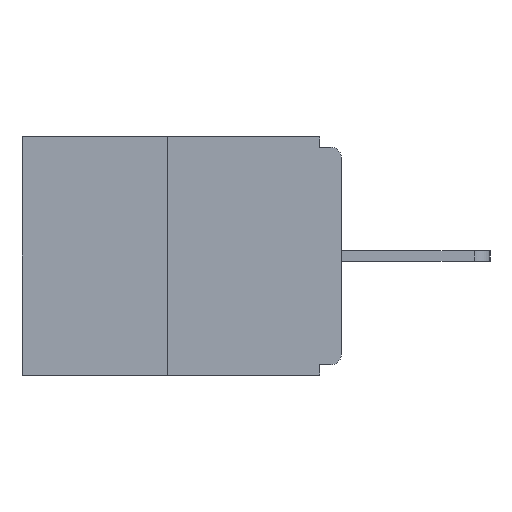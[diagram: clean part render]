
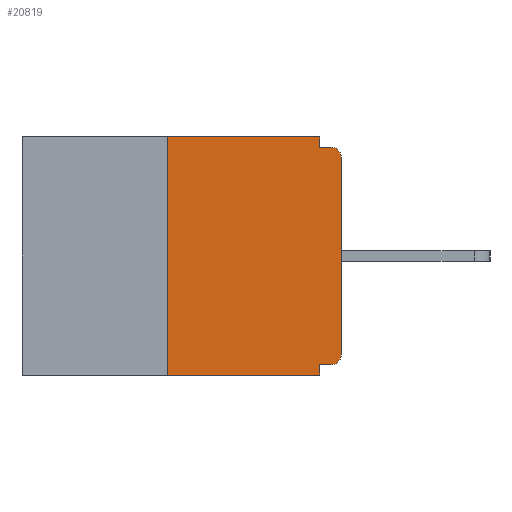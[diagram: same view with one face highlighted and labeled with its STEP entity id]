
A CAD part, left-side view. The second image highlights one B-rep face of the part: STEP entity #20819.
In plain terms, the highlighted planar face has unit normal (-1, 0, 0).
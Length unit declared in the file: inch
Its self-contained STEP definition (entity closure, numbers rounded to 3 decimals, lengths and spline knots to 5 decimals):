
#95 = DIRECTION ( 'NONE',  ( -1., 0., 0. ) ) ;
#302 = EDGE_CURVE ( 'NONE', #7137, #6968, #13642, .T. ) ;
#797 = DIRECTION ( 'NONE',  ( 0., 1., 0. ) ) ;
#963 = ORIENTED_EDGE ( 'NONE', *, *, #16345, .F. ) ;
#1202 = PLANE ( 'NONE',  #10580 ) ;
#1328 = DIRECTION ( 'NONE',  ( 0., 0., -1. ) ) ;
#1522 = CARTESIAN_POINT ( 'NONE',  ( 0., 0.46, 0. ) ) ;
#1648 = VERTEX_POINT ( 'NONE', #4139 ) ;
#1954 = EDGE_CURVE ( 'NONE', #13707, #7137, #19264, .T. ) ;
#2120 = DIRECTION ( 'NONE',  ( 0., -1., 0. ) ) ;
#2138 = VECTOR ( 'NONE', #10817, 39.37008 ) ;
#2271 = CARTESIAN_POINT ( 'NONE',  ( 0., 0.25, 0. ) ) ;
#2463 = CARTESIAN_POINT ( 'NONE',  ( 0., 0.031, 0. ) ) ;
#3085 = DIRECTION ( 'NONE',  ( 0., -1., 0. ) ) ;
#3552 = CARTESIAN_POINT ( 'NONE',  ( 0., 0.46, -0.343 ) ) ;
#3755 = CARTESIAN_POINT ( 'NONE',  ( 0., 0.25, 0. ) ) ;
#4139 = CARTESIAN_POINT ( 'NONE',  ( 0., 0.015, -0.328 ) ) ;
#4356 = DIRECTION ( 'NONE',  ( 0., 0., -1. ) ) ;
#4429 = CARTESIAN_POINT ( 'NONE',  ( 0., 0.031, -0.343 ) ) ;
#4541 = VECTOR ( 'NONE', #20364, 39.37008 ) ;
#4581 = LINE ( 'NONE', #11213, #12436 ) ;
#4691 = CARTESIAN_POINT ( 'NONE',  ( 0., 0.46, 0. ) ) ;
#4740 = AXIS2_PLACEMENT_3D ( 'NONE', #11825, #95, #13228 ) ;
#5364 = ORIENTED_EDGE ( 'NONE', *, *, #1954, .F. ) ;
#5412 = ORIENTED_EDGE ( 'NONE', *, *, #21240, .F. ) ;
#5984 = ORIENTED_EDGE ( 'NONE', *, *, #302, .F. ) ;
#6381 = VERTEX_POINT ( 'NONE', #8549 ) ;
#6968 = VERTEX_POINT ( 'NONE', #12959 ) ;
#7137 = VERTEX_POINT ( 'NONE', #11759 ) ;
#8549 = CARTESIAN_POINT ( 'NONE',  ( 0., 0., -0.03 ) ) ;
#8566 = DIRECTION ( 'NONE',  ( -1., 0., 0. ) ) ;
#8601 = ORIENTED_EDGE ( 'NONE', *, *, #15898, .T. ) ;
#8761 = CARTESIAN_POINT ( 'NONE',  ( 0., 0.031, -0.328 ) ) ;
#8878 = DIRECTION ( 'NONE',  ( 0., 0., 1. ) ) ;
#8931 = CARTESIAN_POINT ( 'NONE',  ( 0., 0., -0.328 ) ) ;
#9085 = CARTESIAN_POINT ( 'NONE',  ( 0., 0., -0.313 ) ) ;
#9409 = CARTESIAN_POINT ( 'NONE',  ( 0., 0., 0. ) ) ;
#9641 = EDGE_CURVE ( 'NONE', #6381, #6968, #14069, .T. ) ;
#9679 = EDGE_CURVE ( 'NONE', #1648, #11336, #13044, .T. ) ;
#9800 = CARTESIAN_POINT ( 'NONE',  ( 0., 0.031, 0. ) ) ;
#9898 = VECTOR ( 'NONE', #16007, 39.37008 ) ;
#9943 = LINE ( 'NONE', #3552, #18592 ) ;
#10031 = EDGE_CURVE ( 'NONE', #11819, #18673, #9943, .T. ) ;
#10580 = AXIS2_PLACEMENT_3D ( 'NONE', #1522, #20942, #4356 ) ;
#10817 = DIRECTION ( 'NONE',  ( 0., 0., 1. ) ) ;
#11213 = CARTESIAN_POINT ( 'NONE',  ( 0., 0.031, -0.343 ) ) ;
#11247 = VERTEX_POINT ( 'NONE', #8761 ) ;
#11336 = VERTEX_POINT ( 'NONE', #9085 ) ;
#11759 = CARTESIAN_POINT ( 'NONE',  ( 0., 0.031, -0.015 ) ) ;
#11819 = VERTEX_POINT ( 'NONE', #14136 ) ;
#11825 = CARTESIAN_POINT ( 'NONE',  ( 0., 0.015, -0.03 ) ) ;
#12436 = VECTOR ( 'NONE', #1328, 39.37008 ) ;
#12959 = CARTESIAN_POINT ( 'NONE',  ( 0., 0.015, -0.015 ) ) ;
#12971 = VECTOR ( 'NONE', #3085, 39.37008 ) ;
#13044 = CIRCLE ( 'NONE', #15822, 0.015 ) ;
#13228 = DIRECTION ( 'NONE',  ( 0., 0., -1. ) ) ;
#13495 = EDGE_LOOP ( 'NONE', ( #16541, #5412, #16545, #14215, #963, #18309, #8601, #16859, #5984, #5364 ) ) ;
#13642 = LINE ( 'NONE', #20262, #4541 ) ;
#13707 = VERTEX_POINT ( 'NONE', #9800 ) ;
#13778 = EDGE_CURVE ( 'NONE', #11247, #18673, #4581, .T. ) ;
#14069 = CIRCLE ( 'NONE', #4740, 0.015 ) ;
#14136 = CARTESIAN_POINT ( 'NONE',  ( 0., 0.25, -0.343 ) ) ;
#14215 = ORIENTED_EDGE ( 'NONE', *, *, #13778, .F. ) ;
#14265 = VECTOR ( 'NONE', #797, 39.37008 ) ;
#15605 = LINE ( 'NONE', #2271, #17277 ) ;
#15822 = AXIS2_PLACEMENT_3D ( 'NONE', #18435, #8566, #21275 ) ;
#15898 = EDGE_CURVE ( 'NONE', #11336, #6381, #18935, .T. ) ;
#16007 = DIRECTION ( 'NONE',  ( 0., 0., -1. ) ) ;
#16345 = EDGE_CURVE ( 'NONE', #1648, #11247, #20423, .T. ) ;
#16541 = ORIENTED_EDGE ( 'NONE', *, *, #20534, .F. ) ;
#16545 = ORIENTED_EDGE ( 'NONE', *, *, #10031, .T. ) ;
#16859 = ORIENTED_EDGE ( 'NONE', *, *, #9641, .T. ) ;
#17277 = VECTOR ( 'NONE', #8878, 39.37008 ) ;
#17450 = VERTEX_POINT ( 'NONE', #3755 ) ;
#18309 = ORIENTED_EDGE ( 'NONE', *, *, #9679, .T. ) ;
#18435 = CARTESIAN_POINT ( 'NONE',  ( 0., 0.015, -0.313 ) ) ;
#18592 = VECTOR ( 'NONE', #2120, 39.37008 ) ;
#18673 = VERTEX_POINT ( 'NONE', #4429 ) ;
#18935 = LINE ( 'NONE', #9409, #2138 ) ;
#19264 = LINE ( 'NONE', #2463, #9898 ) ;
#19560 = LINE ( 'NONE', #4691, #12971 ) ;
#20262 = CARTESIAN_POINT ( 'NONE',  ( 0., 0., -0.015 ) ) ;
#20364 = DIRECTION ( 'NONE',  ( 0., -1., 0. ) ) ;
#20423 = LINE ( 'NONE', #8931, #14265 ) ;
#20534 = EDGE_CURVE ( 'NONE', #17450, #13707, #19560, .T. ) ;
#20613 = FACE_OUTER_BOUND ( 'NONE', #13495, .T. ) ;
#20819 = ADVANCED_FACE ( 'NONE', ( #20613 ), #1202, .F. ) ;
#20942 = DIRECTION ( 'NONE',  ( 1., 0., 0. ) ) ;
#21240 = EDGE_CURVE ( 'NONE', #11819, #17450, #15605, .T. ) ;
#21275 = DIRECTION ( 'NONE',  ( 0., 0., -1. ) ) ;
